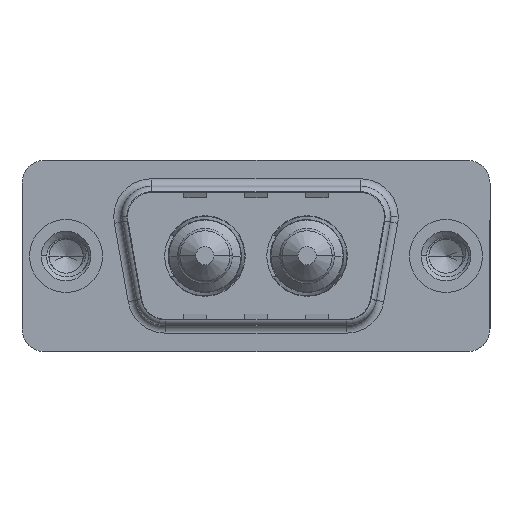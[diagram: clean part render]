
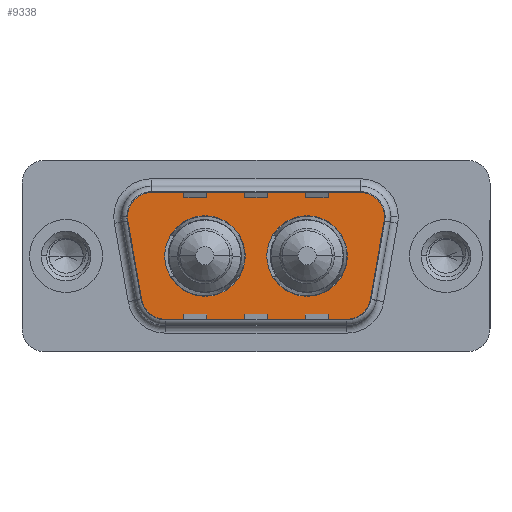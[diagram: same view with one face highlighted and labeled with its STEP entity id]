
A CAD part, top view. The second image highlights one B-rep face of the part: STEP entity #9338.
In plain terms, the highlighted planar face has unit normal (0, 0, 1).
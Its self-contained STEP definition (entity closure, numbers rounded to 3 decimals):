
#59 = LINE ( 'NONE', #10247, #7412 ) ;
#92 = VERTEX_POINT ( 'NONE', #326 ) ;
#138 = CIRCLE ( 'NONE', #11191, 2. ) ;
#267 = DIRECTION ( 'NONE',  ( 1., 0., 0. ) ) ;
#326 = CARTESIAN_POINT ( 'NONE',  ( 5.436, 4.9, 0. ) ) ;
#354 = EDGE_LOOP ( 'NONE', ( #7888, #2601 ) ) ;
#501 = CARTESIAN_POINT ( 'NONE',  ( 6.49, 0., 0. ) ) ;
#599 = CARTESIAN_POINT ( 'NONE',  ( 21.534, 2.553, 0. ) ) ;
#637 = CIRCLE ( 'NONE', #11681, 2.65 ) ;
#660 = EDGE_CURVE ( 'NONE', #3567, #8621, #4387, .T. ) ;
#824 = EDGE_CURVE ( 'NONE', #3630, #8836, #637, .T. ) ;
#1153 = CARTESIAN_POINT ( 'NONE',  ( 11.79, 0., 0. ) ) ;
#1185 = DIRECTION ( 'NONE',  ( -1., 0., 0. ) ) ;
#1215 = CARTESIAN_POINT ( 'NONE',  ( 6.459, -4.9, 0. ) ) ;
#1285 = ORIENTED_EDGE ( 'NONE', *, *, #8380, .T. ) ;
#1417 = DIRECTION ( 'NONE',  ( 0., 0., 1. ) ) ;
#1516 = EDGE_CURVE ( 'NONE', #7808, #92, #10871, .T. ) ;
#1518 = CIRCLE ( 'NONE', #3746, 2. ) ;
#1599 = DIRECTION ( 'NONE',  ( 1., 0., 0. ) ) ;
#1726 = CARTESIAN_POINT ( 'NONE',  ( 5.436, 2.9, 0. ) ) ;
#1757 = CARTESIAN_POINT ( 'NONE',  ( 18.541, -2.9, 0. ) ) ;
#1898 = FACE_OUTER_BOUND ( 'NONE', #11859, .T. ) ;
#2179 = EDGE_CURVE ( 'NONE', #4253, #3300, #6015, .T. ) ;
#2247 = CARTESIAN_POINT ( 'NONE',  ( 3.466, 2.553, 0. ) ) ;
#2338 = ORIENTED_EDGE ( 'NONE', *, *, #7009, .T. ) ;
#2601 = ORIENTED_EDGE ( 'NONE', *, *, #11036, .F. ) ;
#2604 = ORIENTED_EDGE ( 'NONE', *, *, #11304, .T. ) ;
#2690 = DIRECTION ( 'NONE',  ( 1., 0., 0. ) ) ;
#2720 = DIRECTION ( 'NONE',  ( 1., 0., 0. ) ) ;
#3085 = DIRECTION ( 'NONE',  ( 0., 0., 1. ) ) ;
#3100 = AXIS2_PLACEMENT_3D ( 'NONE', #10113, #10070, #10045 ) ;
#3131 = VERTEX_POINT ( 'NONE', #2247 ) ;
#3202 = EDGE_LOOP ( 'NONE', ( #11627, #9641 ) ) ;
#3291 = AXIS2_PLACEMENT_3D ( 'NONE', #6563, #11592, #8095 ) ;
#3300 = VERTEX_POINT ( 'NONE', #7102 ) ;
#3567 = VERTEX_POINT ( 'NONE', #11561 ) ;
#3579 = AXIS2_PLACEMENT_3D ( 'NONE', #8877, #3085, #9838 ) ;
#3630 = VERTEX_POINT ( 'NONE', #1153 ) ;
#3732 = AXIS2_PLACEMENT_3D ( 'NONE', #11024, #1417, #8148 ) ;
#3740 = DIRECTION ( 'NONE',  ( 0.174, 0.985, 0. ) ) ;
#3746 = AXIS2_PLACEMENT_3D ( 'NONE', #9000, #8968, #8955 ) ;
#3942 = EDGE_CURVE ( 'NONE', #7234, #7808, #6394, .T. ) ;
#4083 = DIRECTION ( 'NONE',  ( 0., 0., 1. ) ) ;
#4253 = VERTEX_POINT ( 'NONE', #5461 ) ;
#4277 = PLANE ( 'NONE',  #3732 ) ;
#4387 = CIRCLE ( 'NONE', #3291, 2.65 ) ;
#4438 = ORIENTED_EDGE ( 'NONE', *, *, #2179, .T. ) ;
#4556 = CARTESIAN_POINT ( 'NONE',  ( 5.436, 4.9, 0. ) ) ;
#4888 = CIRCLE ( 'NONE', #7198, 2. ) ;
#5075 = VECTOR ( 'NONE', #267, 1000. ) ;
#5085 = ORIENTED_EDGE ( 'NONE', *, *, #3942, .T. ) ;
#5138 = ORIENTED_EDGE ( 'NONE', *, *, #9208, .T. ) ;
#5308 = ORIENTED_EDGE ( 'NONE', *, *, #6670, .T. ) ;
#5461 = CARTESIAN_POINT ( 'NONE',  ( 20.511, -3.247, 0. ) ) ;
#5591 = ORIENTED_EDGE ( 'NONE', *, *, #7070, .T. ) ;
#5763 = VERTEX_POINT ( 'NONE', #10006 ) ;
#6015 = LINE ( 'NONE', #599, #8588 ) ;
#6209 = VERTEX_POINT ( 'NONE', #8219 ) ;
#6394 = CIRCLE ( 'NONE', #10735, 2. ) ;
#6563 = CARTESIAN_POINT ( 'NONE',  ( 15.86, 0., 0. ) ) ;
#6670 = EDGE_CURVE ( 'NONE', #3131, #5763, #59, .T. ) ;
#7009 = EDGE_CURVE ( 'NONE', #5763, #12377, #12076, .T. ) ;
#7070 = EDGE_CURVE ( 'NONE', #3300, #7234, #1518, .T. ) ;
#7102 = CARTESIAN_POINT ( 'NONE',  ( 21.534, 2.553, 0. ) ) ;
#7198 = AXIS2_PLACEMENT_3D ( 'NONE', #1726, #8456, #2690 ) ;
#7234 = VERTEX_POINT ( 'NONE', #7311 ) ;
#7244 = DIRECTION ( 'NONE',  ( 0., 0., 1. ) ) ;
#7311 = CARTESIAN_POINT ( 'NONE',  ( 21.564, 2.9, 0. ) ) ;
#7320 = CARTESIAN_POINT ( 'NONE',  ( 6.459, -4.9, 0. ) ) ;
#7412 = VECTOR ( 'NONE', #10339, 1000. ) ;
#7743 = ORIENTED_EDGE ( 'NONE', *, *, #1516, .T. ) ;
#7808 = VERTEX_POINT ( 'NONE', #8295 ) ;
#7857 = CARTESIAN_POINT ( 'NONE',  ( 13.21, 0., 0. ) ) ;
#7888 = ORIENTED_EDGE ( 'NONE', *, *, #660, .F. ) ;
#8095 = DIRECTION ( 'NONE',  ( 1., 0., 0. ) ) ;
#8148 = DIRECTION ( 'NONE',  ( 1., 0., 0. ) ) ;
#8219 = CARTESIAN_POINT ( 'NONE',  ( 18.541, -4.9, 0. ) ) ;
#8290 = VECTOR ( 'NONE', #1185, 1000. ) ;
#8291 = CARTESIAN_POINT ( 'NONE',  ( 9.14, 0., 0. ) ) ;
#8295 = CARTESIAN_POINT ( 'NONE',  ( 19.564, 4.9, 0. ) ) ;
#8380 = EDGE_CURVE ( 'NONE', #6209, #4253, #138, .T. ) ;
#8456 = DIRECTION ( 'NONE',  ( 0., 0., 1. ) ) ;
#8496 = DIRECTION ( 'NONE',  ( 0., 0., 1. ) ) ;
#8529 = CIRCLE ( 'NONE', #8846, 2.65 ) ;
#8588 = VECTOR ( 'NONE', #3740, 1000. ) ;
#8621 = VERTEX_POINT ( 'NONE', #7857 ) ;
#8767 = DIRECTION ( 'NONE',  ( -1., 0., 0. ) ) ;
#8836 = VERTEX_POINT ( 'NONE', #501 ) ;
#8846 = AXIS2_PLACEMENT_3D ( 'NONE', #9880, #4083, #10843 ) ;
#8877 = CARTESIAN_POINT ( 'NONE',  ( 15.86, 0., 0. ) ) ;
#8955 = DIRECTION ( 'NONE',  ( -1., 0., 0. ) ) ;
#8968 = DIRECTION ( 'NONE',  ( 0., 0., 1. ) ) ;
#9000 = CARTESIAN_POINT ( 'NONE',  ( 19.564, 2.9, 0. ) ) ;
#9003 = FACE_BOUND ( 'NONE', #354, .T. ) ;
#9208 = EDGE_CURVE ( 'NONE', #12377, #6209, #10518, .T. ) ;
#9338 = ADVANCED_FACE ( 'NONE', ( #9003, #11844, #1898 ), #4277, .T. ) ;
#9641 = ORIENTED_EDGE ( 'NONE', *, *, #10424, .F. ) ;
#9838 = DIRECTION ( 'NONE',  ( 1., 0., 0. ) ) ;
#9880 = CARTESIAN_POINT ( 'NONE',  ( 9.14, 0., 0. ) ) ;
#10006 = CARTESIAN_POINT ( 'NONE',  ( 4.489, -3.247, 0. ) ) ;
#10045 = DIRECTION ( 'NONE',  ( -1., 0., 0. ) ) ;
#10070 = DIRECTION ( 'NONE',  ( 0., 0., 1. ) ) ;
#10113 = CARTESIAN_POINT ( 'NONE',  ( 6.459, -2.9, 0. ) ) ;
#10247 = CARTESIAN_POINT ( 'NONE',  ( 3.466, 2.553, 0. ) ) ;
#10339 = DIRECTION ( 'NONE',  ( 0.174, -0.985, 0. ) ) ;
#10424 = EDGE_CURVE ( 'NONE', #8836, #3630, #8529, .T. ) ;
#10496 = CIRCLE ( 'NONE', #3579, 2.65 ) ;
#10518 = LINE ( 'NONE', #1215, #5075 ) ;
#10735 = AXIS2_PLACEMENT_3D ( 'NONE', #11268, #7244, #8767 ) ;
#10843 = DIRECTION ( 'NONE',  ( 1., 0., 0. ) ) ;
#10871 = LINE ( 'NONE', #4556, #8290 ) ;
#11024 = CARTESIAN_POINT ( 'NONE',  ( 18.541, -2.9, 0. ) ) ;
#11036 = EDGE_CURVE ( 'NONE', #8621, #3567, #10496, .T. ) ;
#11191 = AXIS2_PLACEMENT_3D ( 'NONE', #1757, #8496, #2720 ) ;
#11268 = CARTESIAN_POINT ( 'NONE',  ( 19.564, 2.9, 0. ) ) ;
#11304 = EDGE_CURVE ( 'NONE', #92, #3131, #4888, .T. ) ;
#11561 = CARTESIAN_POINT ( 'NONE',  ( 18.51, 0., 0. ) ) ;
#11592 = DIRECTION ( 'NONE',  ( 0., 0., 1. ) ) ;
#11627 = ORIENTED_EDGE ( 'NONE', *, *, #824, .F. ) ;
#11681 = AXIS2_PLACEMENT_3D ( 'NONE', #8291, #12172, #1599 ) ;
#11844 = FACE_BOUND ( 'NONE', #3202, .T. ) ;
#11859 = EDGE_LOOP ( 'NONE', ( #1285, #4438, #5591, #5085, #7743, #2604, #5308, #2338, #5138 ) ) ;
#12076 = CIRCLE ( 'NONE', #3100, 2. ) ;
#12172 = DIRECTION ( 'NONE',  ( 0., 0., 1. ) ) ;
#12377 = VERTEX_POINT ( 'NONE', #7320 ) ;
